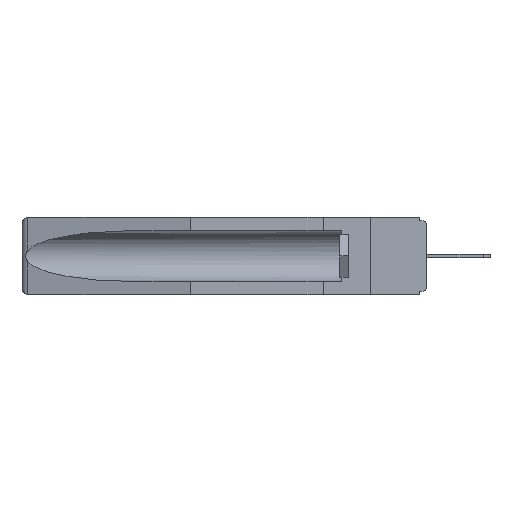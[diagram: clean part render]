
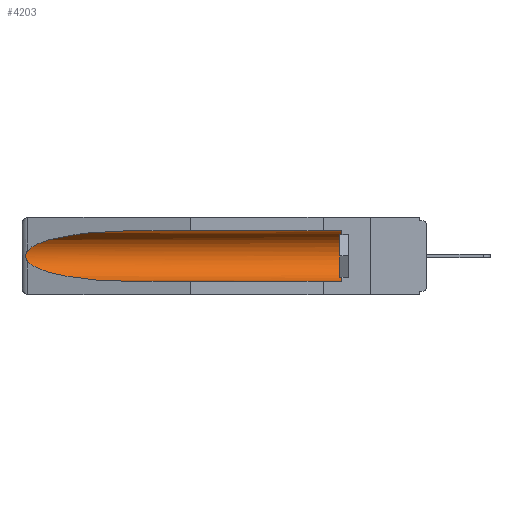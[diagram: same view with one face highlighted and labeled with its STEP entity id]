
A CAD part, left-side view. The second image highlights one B-rep face of the part: STEP entity #4203.
In plain terms, the highlighted cylindrical face has radius 2.857 mm (diameter 5.715 mm), a partial arc.
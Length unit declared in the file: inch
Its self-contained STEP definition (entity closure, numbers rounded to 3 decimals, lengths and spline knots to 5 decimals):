
#25 = VERTEX_POINT ( 'NONE', #15246 ) ;
#120 = CARTESIAN_POINT ( 'NONE',  ( 0.155, 0.126, -0.059 ) ) ;
#241 = AXIS2_PLACEMENT_3D ( 'NONE', #15763, #14692, #15857 ) ;
#1028 = CARTESIAN_POINT ( 'NONE',  ( 0.155, 1.07973, -0.284 ) ) ;
#1173 = CARTESIAN_POINT ( 'NONE',  ( 0.26597, 1.5296, -0.19026 ) ) ;
#1218 = ORIENTED_EDGE ( 'NONE', *, *, #16888, .T. ) ;
#1266 = CARTESIAN_POINT ( 'NONE',  ( 0.2675, 1.53308, -0.16763 ) ) ;
#1388 = CARTESIAN_POINT ( 'NONE',  ( 0.26537, 1.52718, -0.14972 ) ) ;
#1752 = CARTESIAN_POINT ( 'NONE',  ( 0.26537, 1.52718, -0.19328 ) ) ;
#2523 = CARTESIAN_POINT ( 'NONE',  ( 0.26655, 1.53094, -0.18657 ) ) ;
#3001 = EDGE_CURVE ( 'NONE', #14028, #17550, #3126, .T. ) ;
#3126 = B_SPLINE_CURVE_WITH_KNOTS ( 'NONE', 3,
 ( #13455, #14781, #11949, #3938, #1266, #6746, #12211, #2523, #1173, #14613 ),
 .UNSPECIFIED., .F., .F.,
 ( 4, 2, 2, 2, 4 ),
 ( 0., 0.00029, 0.00058, 0.00087, 0.00117 ),
 .UNSPECIFIED. ) ;
#3938 = CARTESIAN_POINT ( 'NONE',  ( 0.2673, 1.5327, -0.16383 ) ) ;
#4008 = VECTOR ( 'NONE', #12833, 39.37008 ) ;
#4203 = ADVANCED_FACE ( 'NONE', ( #15110 ), #13779, .F. ) ;
#4269 = DIRECTION ( 'NONE',  ( 0., 1., 0. ) ) ;
#4636 = ORIENTED_EDGE ( 'NONE', *, *, #12135, .T. ) ;
#5097 = EDGE_CURVE ( 'NONE', #6420, #11100, #17584, .T. ) ;
#5416 = ORIENTED_EDGE ( 'NONE', *, *, #15829, .T. ) ;
#5427 =( BOUNDED_CURVE ( )  B_SPLINE_CURVE ( 3, ( #10659, #16090, #8032, #1388 ),
 .UNSPECIFIED., .F., .T. ) 
 B_SPLINE_CURVE_WITH_KNOTS ( ( 4, 4 ),
 ( 4.71239, 6.08839 ),
 .UNSPECIFIED. ) 
 CURVE ( )  GEOMETRIC_REPRESENTATION_ITEM ( )  RATIONAL_B_SPLINE_CURVE ( ( 1., 0.848, 0.848, 1. ) ) 
 REPRESENTATION_ITEM ( '' )  );
#6420 = VERTEX_POINT ( 'NONE', #10817 ) ;
#6440 = EDGE_LOOP ( 'NONE', ( #5416, #12191, #1218, #15403, #4636, #11250 ) ) ;
#6746 = CARTESIAN_POINT ( 'NONE',  ( 0.2675, 1.53308, -0.17534 ) ) ;
#7244 = CARTESIAN_POINT ( 'NONE',  ( 0.155, 1.07973, -0.284 ) ) ;
#8032 = CARTESIAN_POINT ( 'NONE',  ( 0.25451, 1.48313, -0.09465 ) ) ;
#8071 = CARTESIAN_POINT ( 'NONE',  ( 0.25451, 1.48313, -0.24835 ) ) ;
#8807 = CARTESIAN_POINT ( 'NONE',  ( 0.155, -0.30754, -0.059 ) ) ;
#9404 = CARTESIAN_POINT ( 'NONE',  ( 0.155, -0.30754, -0.1715 ) ) ;
#9453 = CARTESIAN_POINT ( 'NONE',  ( 0.155, -0.30754, -0.284 ) ) ;
#9589 = CARTESIAN_POINT ( 'NONE',  ( 0.26537, 1.52718, -0.14972 ) ) ;
#9974 = AXIS2_PLACEMENT_3D ( 'NONE', #9404, #4269, #12269 ) ;
#10659 = CARTESIAN_POINT ( 'NONE',  ( 0.155, 1.07973, -0.059 ) ) ;
#10817 = CARTESIAN_POINT ( 'NONE',  ( 0.155, 0.126, -0.284 ) ) ;
#11100 = VERTEX_POINT ( 'NONE', #1028 ) ;
#11250 = ORIENTED_EDGE ( 'NONE', *, *, #15245, .T. ) ;
#11949 = CARTESIAN_POINT ( 'NONE',  ( 0.26654, 1.53092, -0.15636 ) ) ;
#12135 = EDGE_CURVE ( 'NONE', #6420, #15009, #13403, .T. ) ;
#12191 = ORIENTED_EDGE ( 'NONE', *, *, #3001, .T. ) ;
#12211 = CARTESIAN_POINT ( 'NONE',  ( 0.2673, 1.53269, -0.17917 ) ) ;
#12269 = DIRECTION ( 'NONE',  ( 0., 0., 1. ) ) ;
#12833 = DIRECTION ( 'NONE',  ( 0., 1., 0. ) ) ;
#13403 = CIRCLE ( 'NONE', #241, 0.1125 ) ;
#13455 = CARTESIAN_POINT ( 'NONE',  ( 0.26537, 1.52718, -0.14972 ) ) ;
#13779 = CYLINDRICAL_SURFACE ( 'NONE', #9974, 0.1125 ) ;
#14028 = VERTEX_POINT ( 'NONE', #9589 ) ;
#14124 = CARTESIAN_POINT ( 'NONE',  ( 0.21114, 1.30732, -0.284 ) ) ;
#14576 =( BOUNDED_CURVE ( )  B_SPLINE_CURVE ( 3, ( #1752, #8071, #14124, #7244 ),
 .UNSPECIFIED., .F., .F. ) 
 B_SPLINE_CURVE_WITH_KNOTS ( ( 4, 4 ),
 ( 0.1948, 1.5708 ),
 .UNSPECIFIED. ) 
 CURVE ( )  GEOMETRIC_REPRESENTATION_ITEM ( )  RATIONAL_B_SPLINE_CURVE ( ( 1., 0.848, 0.848, 1. ) ) 
 REPRESENTATION_ITEM ( '' )  );
#14613 = CARTESIAN_POINT ( 'NONE',  ( 0.26537, 1.52718, -0.19328 ) ) ;
#14692 = DIRECTION ( 'NONE',  ( 0., -1., 0. ) ) ;
#14781 = CARTESIAN_POINT ( 'NONE',  ( 0.26597, 1.52961, -0.15275 ) ) ;
#15009 = VERTEX_POINT ( 'NONE', #120 ) ;
#15110 = FACE_OUTER_BOUND ( 'NONE', #6440, .T. ) ;
#15245 = EDGE_CURVE ( 'NONE', #15009, #25, #17196, .T. ) ;
#15246 = CARTESIAN_POINT ( 'NONE',  ( 0.155, 1.07973, -0.059 ) ) ;
#15302 = VECTOR ( 'NONE', #16430, 39.37008 ) ;
#15403 = ORIENTED_EDGE ( 'NONE', *, *, #5097, .F. ) ;
#15763 = CARTESIAN_POINT ( 'NONE',  ( 0.155, 0.126, -0.1715 ) ) ;
#15829 = EDGE_CURVE ( 'NONE', #25, #14028, #5427, .T. ) ;
#15857 = DIRECTION ( 'NONE',  ( 0., 0., 1. ) ) ;
#16090 = CARTESIAN_POINT ( 'NONE',  ( 0.21114, 1.30732, -0.059 ) ) ;
#16430 = DIRECTION ( 'NONE',  ( 0., 1., 0. ) ) ;
#16888 = EDGE_CURVE ( 'NONE', #17550, #11100, #14576, .T. ) ;
#17196 = LINE ( 'NONE', #8807, #4008 ) ;
#17376 = CARTESIAN_POINT ( 'NONE',  ( 0.26537, 1.52718, -0.19328 ) ) ;
#17550 = VERTEX_POINT ( 'NONE', #17376 ) ;
#17584 = LINE ( 'NONE', #9453, #15302 ) ;
